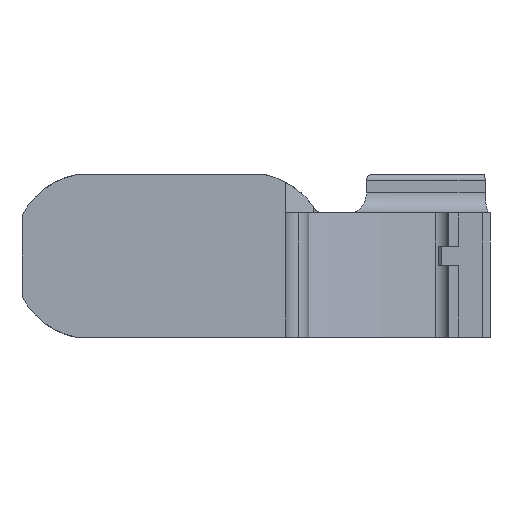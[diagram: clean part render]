
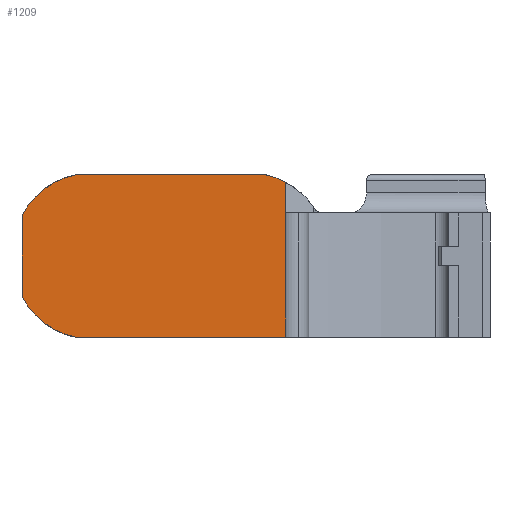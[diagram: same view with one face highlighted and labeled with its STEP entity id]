
A CAD part, front view. The second image highlights one B-rep face of the part: STEP entity #1209.
In plain terms, the highlighted planar face has unit normal (0, -1, 0).
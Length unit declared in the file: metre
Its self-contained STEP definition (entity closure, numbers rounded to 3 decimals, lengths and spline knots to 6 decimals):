
#60=PLANE('',#1342);
#112=FACE_OUTER_BOUND('',#175,.T.);
#175=EDGE_LOOP('',(#1037,#1038,#1039,#1040,#1041,#1042,#1043));
#199=LINE('',#1745,#318);
#226=LINE('',#1843,#345);
#294=LINE('',#2038,#413);
#295=LINE('',#2041,#414);
#318=VECTOR('',#1387,0.014606);
#345=VECTOR('',#1468,0.016179);
#413=VECTOR('',#1656,0.006173);
#414=VECTOR('',#1659,0.011874);
#472=CIRCLE('',#1343,0.005934);
#473=CIRCLE('',#1344,0.005934);
#474=CIRCLE('',#1345,0.005934);
#485=VERTEX_POINT('',#1742);
#486=VERTEX_POINT('',#1744);
#529=VERTEX_POINT('',#1840);
#530=VERTEX_POINT('',#1842);
#582=VERTEX_POINT('',#2035);
#583=VERTEX_POINT('',#2037);
#584=VERTEX_POINT('',#2040);
#605=EDGE_CURVE('',#485,#486,#199,.T.);
#654=EDGE_CURVE('',#530,#529,#226,.T.);
#745=EDGE_CURVE('',#485,#582,#472,.F.);
#746=EDGE_CURVE('',#582,#583,#294,.T.);
#747=EDGE_CURVE('',#583,#530,#473,.F.);
#748=EDGE_CURVE('',#584,#529,#295,.T.);
#749=EDGE_CURVE('',#486,#584,#474,.T.);
#1037=ORIENTED_EDGE('',*,*,#605,.F.);
#1038=ORIENTED_EDGE('',*,*,#745,.T.);
#1039=ORIENTED_EDGE('',*,*,#746,.T.);
#1040=ORIENTED_EDGE('',*,*,#747,.T.);
#1041=ORIENTED_EDGE('',*,*,#654,.T.);
#1042=ORIENTED_EDGE('',*,*,#748,.F.);
#1043=ORIENTED_EDGE('',*,*,#749,.F.);
#1209=ADVANCED_FACE('',(#112),#60,.F.);
#1342=AXIS2_PLACEMENT_3D('',#2034,#1652,#1653);
#1343=AXIS2_PLACEMENT_3D('',#2036,#1654,#1655);
#1344=AXIS2_PLACEMENT_3D('',#2039,#1657,#1658);
#1345=AXIS2_PLACEMENT_3D('',#2042,#1660,#1661);
#1387=DIRECTION('',(1.,0.,0.));
#1468=DIRECTION('',(1.,0.,0.));
#1652=DIRECTION('center_axis',(0.,1.,0.));
#1653=DIRECTION('ref_axis',(-1.,0.,0.));
#1654=DIRECTION('center_axis',(0.,1.,0.));
#1655=DIRECTION('ref_axis',(-1.,0.,0.));
#1656=DIRECTION('',(0.,0.,-1.));
#1657=DIRECTION('center_axis',(0.,1.,0.));
#1658=DIRECTION('ref_axis',(-1.,0.,0.));
#1659=DIRECTION('',(0.,0.,-1.));
#1660=DIRECTION('center_axis',(0.,1.,0.));
#1661=DIRECTION('ref_axis',(-1.,0.,0.));
#1742=CARTESIAN_POINT('',(-0.00605,-0.009525,0.00562));
#1744=CARTESIAN_POINT('',(0.008555,-0.009525,0.00562));
#1745=CARTESIAN_POINT('',(-0.00605,-0.009525,0.00562));
#1840=CARTESIAN_POINT('',(0.010128,-0.009525,-0.006826));
#1842=CARTESIAN_POINT('',(-0.00605,-0.009525,-0.006826));
#1843=CARTESIAN_POINT('',(-0.00605,-0.009525,-0.006826));
#2034=CARTESIAN_POINT('Origin',(-0.000603,-0.009525,0.00562));
#2035=CARTESIAN_POINT('',(-0.010128,-0.009525,0.002483));
#2036=CARTESIAN_POINT('Origin',(-0.004829,-0.009525,-0.000187));
#2037=CARTESIAN_POINT('',(-0.010128,-0.009525,-0.00369));
#2038=CARTESIAN_POINT('',(-0.010128,-0.009525,0.002483));
#2039=CARTESIAN_POINT('Origin',(-0.004829,-0.009525,-0.001019));
#2040=CARTESIAN_POINT('',(0.010128,-0.009525,0.005048));
#2041=CARTESIAN_POINT('',(0.010128,-0.009525,0.005048));
#2042=CARTESIAN_POINT('Origin',(0.007334,-0.009525,-0.000187));
